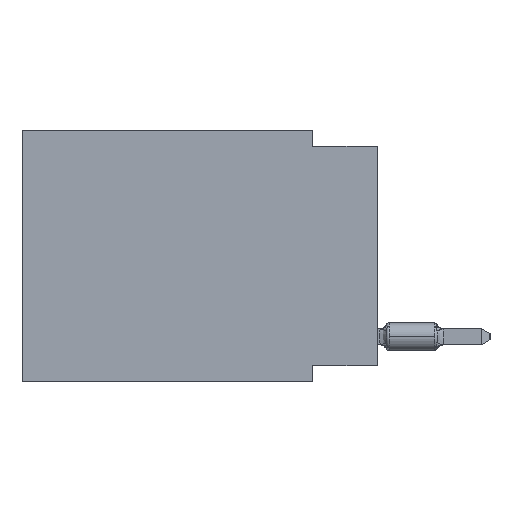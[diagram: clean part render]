
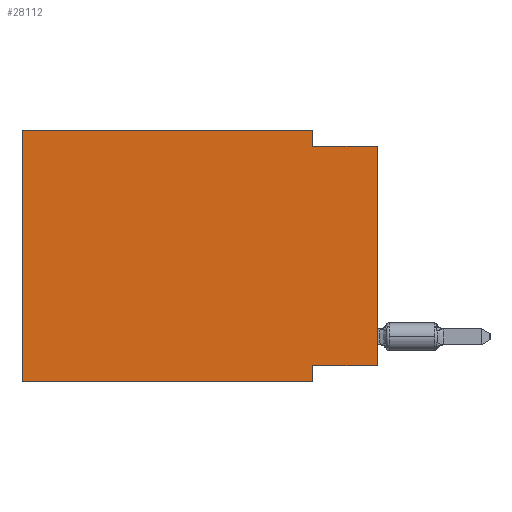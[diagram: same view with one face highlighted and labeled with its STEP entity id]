
A CAD part, left-side view. The second image highlights one B-rep face of the part: STEP entity #28112.
In plain terms, the highlighted planar face has unit normal (-1, 0, 0).
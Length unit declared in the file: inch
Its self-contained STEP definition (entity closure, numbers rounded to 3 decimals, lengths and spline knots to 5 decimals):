
#342 = CARTESIAN_POINT ( 'NONE',  ( 0., 0.1, -0.39 ) ) ;
#664 = VERTEX_POINT ( 'NONE', #8333 ) ;
#1804 = LINE ( 'NONE', #18925, #13794 ) ;
#1867 = ORIENTED_EDGE ( 'NONE', *, *, #11544, .T. ) ;
#2069 = ORIENTED_EDGE ( 'NONE', *, *, #12928, .F. ) ;
#2360 = LINE ( 'NONE', #14024, #25797 ) ;
#2424 = LINE ( 'NONE', #22636, #2979 ) ;
#2756 = VERTEX_POINT ( 'NONE', #8758 ) ;
#2775 = DIRECTION ( 'NONE',  ( 0., 0., -1. ) ) ;
#2950 = ORIENTED_EDGE ( 'NONE', *, *, #19428, .T. ) ;
#2979 = VECTOR ( 'NONE', #15029, 39.37008 ) ;
#3453 = LINE ( 'NONE', #8156, #14145 ) ;
#3848 = VECTOR ( 'NONE', #28115, 39.37008 ) ;
#4277 = EDGE_CURVE ( 'NONE', #21730, #24528, #3453, .T. ) ;
#5056 = PLANE ( 'NONE',  #19195 ) ;
#5493 = CARTESIAN_POINT ( 'NONE',  ( 0., 0.55, -0.39 ) ) ;
#6183 = CARTESIAN_POINT ( 'NONE',  ( 0., 0., -0.025 ) ) ;
#6336 = DIRECTION ( 'NONE',  ( 0., -1., 0. ) ) ;
#7734 = CARTESIAN_POINT ( 'NONE',  ( 0., 0.1, -0.025 ) ) ;
#8156 = CARTESIAN_POINT ( 'NONE',  ( 0., 0.55, 0. ) ) ;
#8333 = CARTESIAN_POINT ( 'NONE',  ( 0., 0.1, -0.365 ) ) ;
#8758 = CARTESIAN_POINT ( 'NONE',  ( 0., 0., -0.025 ) ) ;
#8840 = ORIENTED_EDGE ( 'NONE', *, *, #26942, .F. ) ;
#8915 = CARTESIAN_POINT ( 'NONE',  ( 0., 0.1, 0. ) ) ;
#10377 = CARTESIAN_POINT ( 'NONE',  ( 0., 0.55, 0. ) ) ;
#10488 = DIRECTION ( 'NONE',  ( 0., 1., 0. ) ) ;
#10934 = LINE ( 'NONE', #15489, #15513 ) ;
#11544 = EDGE_CURVE ( 'NONE', #23585, #2756, #2424, .T. ) ;
#11792 = VECTOR ( 'NONE', #26399, 39.37008 ) ;
#12003 = VERTEX_POINT ( 'NONE', #7734 ) ;
#12928 = EDGE_CURVE ( 'NONE', #24528, #12003, #13233, .T. ) ;
#13233 = LINE ( 'NONE', #30862, #3848 ) ;
#13794 = VECTOR ( 'NONE', #15866, 39.37008 ) ;
#13812 = EDGE_LOOP ( 'NONE', ( #1867, #23292, #2069, #25614, #28542, #2950, #30190, #8840 ) ) ;
#14024 = CARTESIAN_POINT ( 'NONE',  ( 0., 0.1, -0.39 ) ) ;
#14145 = VECTOR ( 'NONE', #15261, 39.37008 ) ;
#15029 = DIRECTION ( 'NONE',  ( 0., 0., 1. ) ) ;
#15261 = DIRECTION ( 'NONE',  ( 0., -1., 0. ) ) ;
#15489 = CARTESIAN_POINT ( 'NONE',  ( 0., 0., -0.365 ) ) ;
#15513 = VECTOR ( 'NONE', #10488, 39.37008 ) ;
#15866 = DIRECTION ( 'NONE',  ( 0., 0., 1. ) ) ;
#16404 = EDGE_CURVE ( 'NONE', #23411, #21730, #1804, .T. ) ;
#16460 = EDGE_CURVE ( 'NONE', #12003, #2756, #26373, .T. ) ;
#16523 = CARTESIAN_POINT ( 'NONE',  ( 0., 0.55, -0.39 ) ) ;
#17950 = VECTOR ( 'NONE', #6336, 39.37008 ) ;
#18925 = CARTESIAN_POINT ( 'NONE',  ( 0., 0.55, 0. ) ) ;
#18951 = LINE ( 'NONE', #16523, #11792 ) ;
#19195 = AXIS2_PLACEMENT_3D ( 'NONE', #10377, #20537, #2775 ) ;
#19428 = EDGE_CURVE ( 'NONE', #23411, #20001, #18951, .T. ) ;
#20001 = VERTEX_POINT ( 'NONE', #342 ) ;
#20272 = EDGE_CURVE ( 'NONE', #664, #20001, #2360, .T. ) ;
#20537 = DIRECTION ( 'NONE',  ( 1., 0., 0. ) ) ;
#21730 = VERTEX_POINT ( 'NONE', #22653 ) ;
#22076 = DIRECTION ( 'NONE',  ( 0., 0., -1. ) ) ;
#22636 = CARTESIAN_POINT ( 'NONE',  ( 0., 0., 0. ) ) ;
#22653 = CARTESIAN_POINT ( 'NONE',  ( 0., 0.55, 0. ) ) ;
#23292 = ORIENTED_EDGE ( 'NONE', *, *, #16460, .F. ) ;
#23411 = VERTEX_POINT ( 'NONE', #5493 ) ;
#23585 = VERTEX_POINT ( 'NONE', #23700 ) ;
#23700 = CARTESIAN_POINT ( 'NONE',  ( 0., 0., -0.365 ) ) ;
#24436 = FACE_OUTER_BOUND ( 'NONE', #13812, .T. ) ;
#24528 = VERTEX_POINT ( 'NONE', #8915 ) ;
#25614 = ORIENTED_EDGE ( 'NONE', *, *, #4277, .F. ) ;
#25797 = VECTOR ( 'NONE', #22076, 39.37008 ) ;
#26373 = LINE ( 'NONE', #6183, #17950 ) ;
#26399 = DIRECTION ( 'NONE',  ( 0., -1., 0. ) ) ;
#26942 = EDGE_CURVE ( 'NONE', #23585, #664, #10934, .T. ) ;
#28112 = ADVANCED_FACE ( 'NONE', ( #24436 ), #5056, .F. ) ;
#28115 = DIRECTION ( 'NONE',  ( 0., 0., -1. ) ) ;
#28542 = ORIENTED_EDGE ( 'NONE', *, *, #16404, .F. ) ;
#30190 = ORIENTED_EDGE ( 'NONE', *, *, #20272, .F. ) ;
#30862 = CARTESIAN_POINT ( 'NONE',  ( 0., 0.1, 0. ) ) ;
